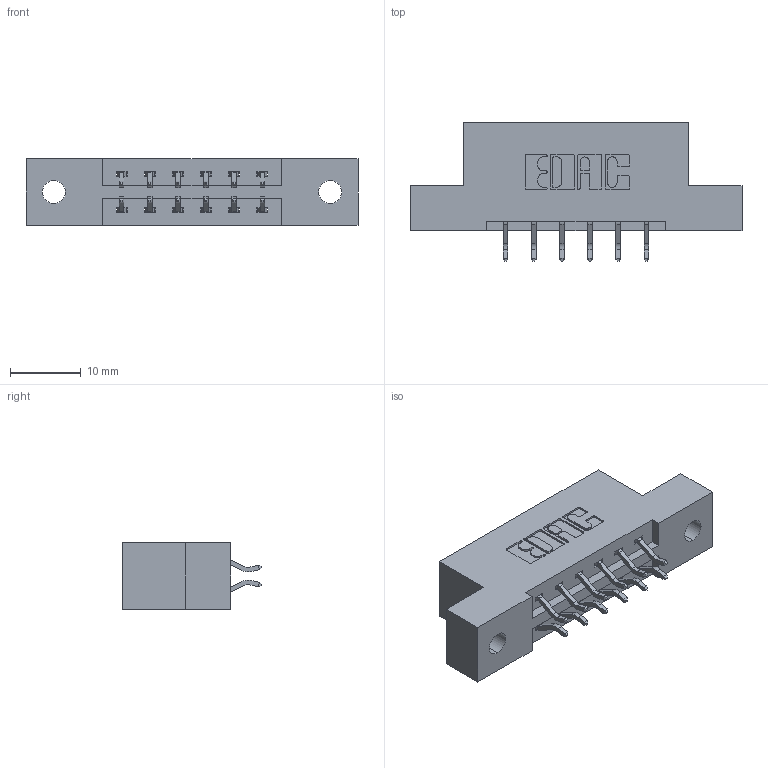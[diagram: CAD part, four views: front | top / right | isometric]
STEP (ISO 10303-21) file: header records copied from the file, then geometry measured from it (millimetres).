
FILE_DESCRIPTION (( 'STEP AP203' ), '1' );
FILE_NAME ('337-012-556-202.STEP', '2018-08-04T05:13:26', ( '' ), ( '' ), 'SwSTEP 2.0', 'SolidWorks 2016', '' );
FILE_SCHEMA (( 'CONFIG_CONTROL_DESIGN' ));
Length unit declared in the file: inch
Products named in the file (3): 337-012-556-202; 345-292-001_556 Tail; 337 Part_Flush Mounting Lugs - 0.128 Dia
Assembly tree (13 placements, depth 2):
  337-012-556-202
    337 Part_Flush Mounting Lugs - 0.128 Dia
    345-292-001_556 Tail  x12
Bounding box: 46.79 x 19.57 x 9.4 mm (x, y, z)
Volume: 4414.4 mm3; surface area: 4355.4 mm2
Topology: 13 solids, 13 shells, 834 faces, 2459 edges, 1622 vertices
Faces by surface type: plane 574, cylinder 260
Entity records: 9531 total; most frequent: CARTESIAN_POINT 1650, ORIENTED_EDGE 1574, DIRECTION 1459, EDGE_CURVE 787, VECTOR 651, LINE 651, VERTEX_POINT 522, AXIS2_PLACEMENT_3D 404
